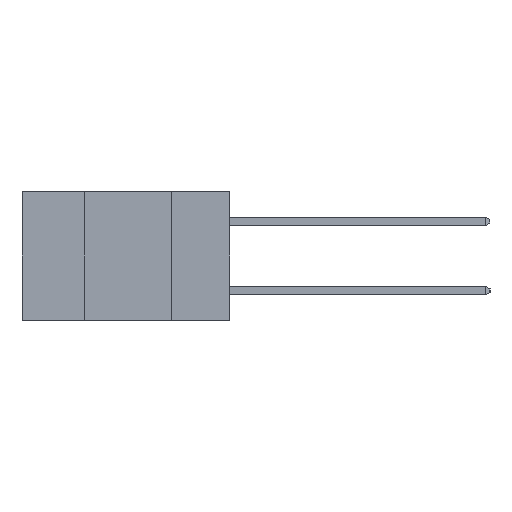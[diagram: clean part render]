
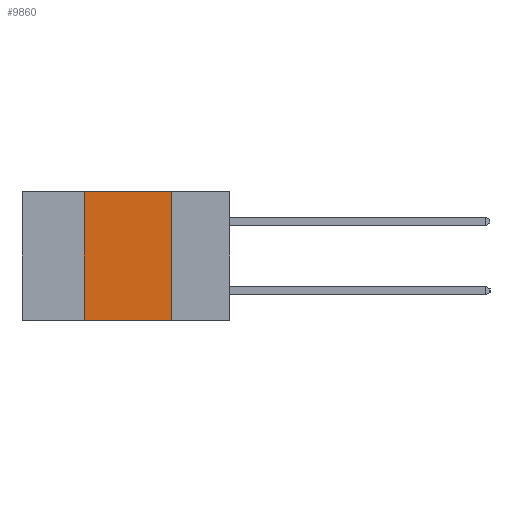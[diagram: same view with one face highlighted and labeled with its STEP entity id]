
A CAD part, left-side view. The second image highlights one B-rep face of the part: STEP entity #9860.
In plain terms, the highlighted planar face has unit normal (-1, 0, 0).
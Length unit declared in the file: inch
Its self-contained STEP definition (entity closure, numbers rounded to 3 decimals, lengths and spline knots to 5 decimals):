
#45 = EDGE_CURVE ( 'NONE', #6744, #5376, #18264, .T. ) ;
#73 = CARTESIAN_POINT ( 'NONE',  ( 0., 0.6, -0.37 ) ) ;
#131 = DIRECTION ( 'NONE',  ( 0., -1., 0. ) ) ;
#1940 = LINE ( 'NONE', #73, #5711 ) ;
#3714 = EDGE_CURVE ( 'NONE', #15353, #19440, #18873, .T. ) ;
#3865 = ORIENTED_EDGE ( 'NONE', *, *, #10810, .T. ) ;
#3939 = LINE ( 'NONE', #5698, #4436 ) ;
#4100 = DIRECTION ( 'NONE',  ( 0., 0., -1. ) ) ;
#4394 = CARTESIAN_POINT ( 'NONE',  ( 0., 0.42, -0.37 ) ) ;
#4436 = VECTOR ( 'NONE', #16834, 39.37008 ) ;
#5094 = VECTOR ( 'NONE', #14076, 39.37008 ) ;
#5371 = ORIENTED_EDGE ( 'NONE', *, *, #16547, .F. ) ;
#5376 = VERTEX_POINT ( 'NONE', #18474 ) ;
#5587 = DIRECTION ( 'NONE',  ( 0., 0., -1. ) ) ;
#5667 = CARTESIAN_POINT ( 'NONE',  ( 0., 0.17, 0. ) ) ;
#5698 = CARTESIAN_POINT ( 'NONE',  ( 0., 0.6, 0. ) ) ;
#5711 = VECTOR ( 'NONE', #131, 39.37008 ) ;
#5998 = DIRECTION ( 'NONE',  ( 1., 0., 0. ) ) ;
#6215 = VECTOR ( 'NONE', #4100, 39.37008 ) ;
#6283 = CARTESIAN_POINT ( 'NONE',  ( 0., 0.6, 0. ) ) ;
#6744 = VERTEX_POINT ( 'NONE', #15694 ) ;
#7160 = CARTESIAN_POINT ( 'NONE',  ( 0., 0.17, -0.37 ) ) ;
#7849 = PLANE ( 'NONE',  #18751 ) ;
#9632 = ORIENTED_EDGE ( 'NONE', *, *, #3714, .F. ) ;
#9637 = CARTESIAN_POINT ( 'NONE',  ( 0., 0.17, -0.37 ) ) ;
#9860 = ADVANCED_FACE ( 'NONE', ( #15744 ), #7849, .F. ) ;
#10810 = EDGE_CURVE ( 'NONE', #6744, #19440, #1940, .T. ) ;
#13412 = ORIENTED_EDGE ( 'NONE', *, *, #45, .F. ) ;
#14076 = DIRECTION ( 'NONE',  ( 0., 0., 1. ) ) ;
#14885 = EDGE_LOOP ( 'NONE', ( #9632, #5371, #13412, #3865 ) ) ;
#15353 = VERTEX_POINT ( 'NONE', #5667 ) ;
#15694 = CARTESIAN_POINT ( 'NONE',  ( 0., 0.42, -0.37 ) ) ;
#15744 = FACE_OUTER_BOUND ( 'NONE', #14885, .T. ) ;
#16547 = EDGE_CURVE ( 'NONE', #5376, #15353, #3939, .T. ) ;
#16834 = DIRECTION ( 'NONE',  ( 0., -1., 0. ) ) ;
#18264 = LINE ( 'NONE', #4394, #5094 ) ;
#18474 = CARTESIAN_POINT ( 'NONE',  ( 0., 0.42, 0. ) ) ;
#18751 = AXIS2_PLACEMENT_3D ( 'NONE', #6283, #5998, #5587 ) ;
#18873 = LINE ( 'NONE', #9637, #6215 ) ;
#19440 = VERTEX_POINT ( 'NONE', #7160 ) ;
